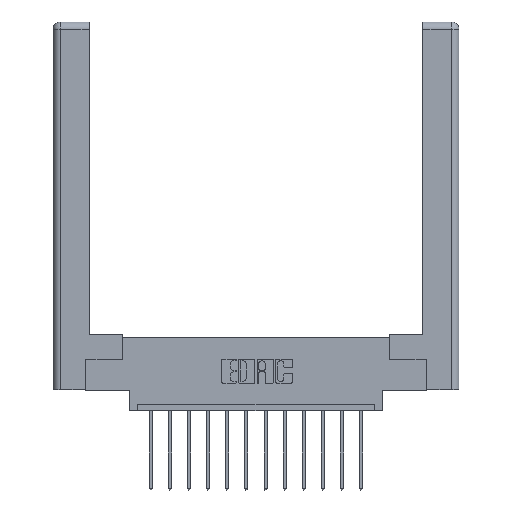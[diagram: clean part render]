
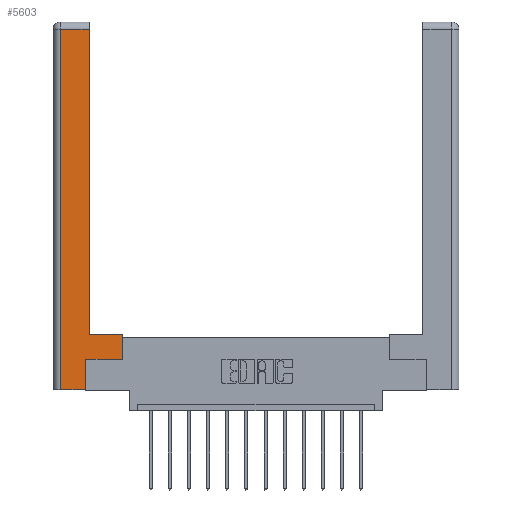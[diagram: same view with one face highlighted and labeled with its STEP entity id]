
A CAD part, top view. The second image highlights one B-rep face of the part: STEP entity #5603.
In plain terms, the highlighted planar face has unit normal (0, 0, 1).
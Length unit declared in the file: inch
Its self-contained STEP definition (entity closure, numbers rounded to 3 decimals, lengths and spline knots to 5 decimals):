
#401 = LINE ( 'NONE', #1041, #5844 ) ;
#531 = DIRECTION ( 'NONE',  ( 0., 1., 0. ) ) ;
#554 = EDGE_CURVE ( 'NONE', #6870, #8590, #12276, .T. ) ;
#909 = PLANE ( 'NONE',  #3713 ) ;
#1041 = CARTESIAN_POINT ( 'NONE',  ( 0.0615, 0., 0. ) ) ;
#1149 = DIRECTION ( 'NONE',  ( 1., 0., 0. ) ) ;
#1542 = EDGE_CURVE ( 'NONE', #6187, #4255, #11482, .T. ) ;
#1637 = DIRECTION ( 'NONE',  ( 0., 1., 0. ) ) ;
#1664 = CARTESIAN_POINT ( 'NONE',  ( 0.295, 0.45, 0. ) ) ;
#2158 = CARTESIAN_POINT ( 'NONE',  ( 0., 0., 0. ) ) ;
#2249 = ORIENTED_EDGE ( 'NONE', *, *, #13947, .T. ) ;
#2559 = EDGE_CURVE ( 'NONE', #5593, #2609, #9027, .T. ) ;
#2609 = VERTEX_POINT ( 'NONE', #11502 ) ;
#2814 = CARTESIAN_POINT ( 'NONE',  ( 0.295, 3., 0. ) ) ;
#3355 = DIRECTION ( 'NONE',  ( -1., 0., 0. ) ) ;
#3545 = LINE ( 'NONE', #8148, #15374 ) ;
#3551 = DIRECTION ( 'NONE',  ( 0., -1., 0. ) ) ;
#3686 = CARTESIAN_POINT ( 'NONE',  ( 0.265, 0.245, 0. ) ) ;
#3713 = AXIS2_PLACEMENT_3D ( 'NONE', #2158, #10508, #3355 ) ;
#4255 = VERTEX_POINT ( 'NONE', #6972 ) ;
#4793 = VECTOR ( 'NONE', #1149, 39.37008 ) ;
#4838 = ORIENTED_EDGE ( 'NONE', *, *, #10183, .T. ) ;
#5120 = VECTOR ( 'NONE', #11424, 39.37008 ) ;
#5125 = EDGE_LOOP ( 'NONE', ( #2249, #14729, #11546, #13060, #14282, #4838, #11111, #7927 ) ) ;
#5427 = VECTOR ( 'NONE', #13251, 39.37008 ) ;
#5544 = EDGE_CURVE ( 'NONE', #4255, #7452, #3545, .T. ) ;
#5593 = VERTEX_POINT ( 'NONE', #15269 ) ;
#5603 = ADVANCED_FACE ( 'NONE', ( #9119 ), #909, .F. ) ;
#5725 = DIRECTION ( 'NONE',  ( -1., 0., 0. ) ) ;
#5844 = VECTOR ( 'NONE', #3551, 39.37008 ) ;
#6187 = VERTEX_POINT ( 'NONE', #9602 ) ;
#6870 = VERTEX_POINT ( 'NONE', #11280 ) ;
#6943 = LINE ( 'NONE', #13689, #12370 ) ;
#6972 = CARTESIAN_POINT ( 'NONE',  ( 0.565, 0.45, 0. ) ) ;
#7240 = CARTESIAN_POINT ( 'NONE',  ( 0.265, 0., 0. ) ) ;
#7310 = LINE ( 'NONE', #3686, #5427 ) ;
#7452 = VERTEX_POINT ( 'NONE', #1664 ) ;
#7638 = VERTEX_POINT ( 'NONE', #8145 ) ;
#7927 = ORIENTED_EDGE ( 'NONE', *, *, #5544, .T. ) ;
#7951 = VECTOR ( 'NONE', #1637, 39.37008 ) ;
#8145 = CARTESIAN_POINT ( 'NONE',  ( 0.265, 0.245, 0. ) ) ;
#8148 = CARTESIAN_POINT ( 'NONE',  ( 0.295, 0.45, 0. ) ) ;
#8183 = EDGE_CURVE ( 'NONE', #2609, #6870, #401, .T. ) ;
#8472 = VECTOR ( 'NONE', #531, 39.37008 ) ;
#8590 = VERTEX_POINT ( 'NONE', #14180 ) ;
#9027 = LINE ( 'NONE', #9099, #5120 ) ;
#9099 = CARTESIAN_POINT ( 'NONE',  ( 0.0615, 2.94, 0. ) ) ;
#9119 = FACE_OUTER_BOUND ( 'NONE', #5125, .T. ) ;
#9602 = CARTESIAN_POINT ( 'NONE',  ( 0.565, 0.245, 0. ) ) ;
#10074 = CARTESIAN_POINT ( 'NONE',  ( 0.565, 0.45, 0. ) ) ;
#10183 = EDGE_CURVE ( 'NONE', #7638, #6187, #6943, .T. ) ;
#10508 = DIRECTION ( 'NONE',  ( 0., 0., -1. ) ) ;
#10526 = EDGE_CURVE ( 'NONE', #8590, #7638, #7310, .T. ) ;
#11111 = ORIENTED_EDGE ( 'NONE', *, *, #1542, .T. ) ;
#11280 = CARTESIAN_POINT ( 'NONE',  ( 0.0615, 0., 0. ) ) ;
#11424 = DIRECTION ( 'NONE',  ( -1., 0., 0. ) ) ;
#11482 = LINE ( 'NONE', #10074, #8472 ) ;
#11502 = CARTESIAN_POINT ( 'NONE',  ( 0.0615, 2.94, 0. ) ) ;
#11546 = ORIENTED_EDGE ( 'NONE', *, *, #8183, .T. ) ;
#12275 = LINE ( 'NONE', #2814, #7951 ) ;
#12276 = LINE ( 'NONE', #7240, #4793 ) ;
#12370 = VECTOR ( 'NONE', #15373, 39.37008 ) ;
#13060 = ORIENTED_EDGE ( 'NONE', *, *, #554, .T. ) ;
#13251 = DIRECTION ( 'NONE',  ( 0., 1., 0. ) ) ;
#13689 = CARTESIAN_POINT ( 'NONE',  ( 0.565, 0.245, 0. ) ) ;
#13947 = EDGE_CURVE ( 'NONE', #7452, #5593, #12275, .T. ) ;
#14180 = CARTESIAN_POINT ( 'NONE',  ( 0.265, 0., 0. ) ) ;
#14282 = ORIENTED_EDGE ( 'NONE', *, *, #10526, .T. ) ;
#14729 = ORIENTED_EDGE ( 'NONE', *, *, #2559, .T. ) ;
#15269 = CARTESIAN_POINT ( 'NONE',  ( 0.295, 2.94, 0. ) ) ;
#15373 = DIRECTION ( 'NONE',  ( 1., 0., 0. ) ) ;
#15374 = VECTOR ( 'NONE', #5725, 39.37008 ) ;
